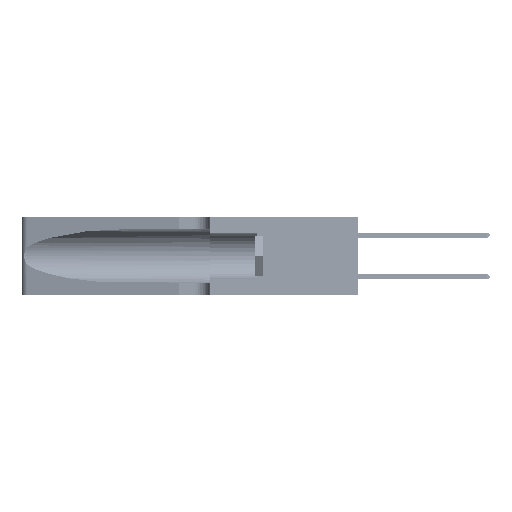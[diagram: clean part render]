
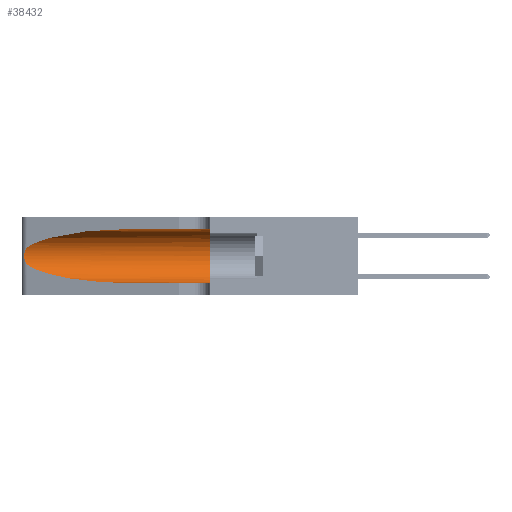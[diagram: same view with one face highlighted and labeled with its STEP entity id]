
A CAD part, left-side view. The second image highlights one B-rep face of the part: STEP entity #38432.
In plain terms, the highlighted cylindrical face has radius 3.308 mm (diameter 6.617 mm), a partial arc.
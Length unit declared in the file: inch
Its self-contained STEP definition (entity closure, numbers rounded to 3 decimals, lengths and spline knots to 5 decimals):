
#1168 = ORIENTED_EDGE ( 'NONE', *, *, #25749, .F. ) ;
#1344 = ORIENTED_EDGE ( 'NONE', *, *, #44045, .T. ) ;
#1497 = CARTESIAN_POINT ( 'NONE',  ( 0.1305, 0.35, 0.185 ) ) ;
#2824 = VERTEX_POINT ( 'NONE', #26665 ) ;
#3456 = CARTESIAN_POINT ( 'NONE',  ( 0.26075, 1.23896, 0.19203 ) ) ;
#3629 = CARTESIAN_POINT ( 'NONE',  ( 0.25487, 1.22718, 0.14631 ) ) ;
#4826 = VERTEX_POINT ( 'NONE', #18742 ) ;
#5212 = CARTESIAN_POINT ( 'NONE',  ( 0.1305, 1.61858, 0.05475 ) ) ;
#5369 = CARTESIAN_POINT ( 'NONE',  ( 0.1305, 0.72297, 0.31525 ) ) ;
#5439 = ORIENTED_EDGE ( 'NONE', *, *, #52243, .T. ) ;
#5553 = CARTESIAN_POINT ( 'NONE',  ( 0.25487, 1.22718, 0.22369 ) ) ;
#5779 = DIRECTION ( 'NONE',  ( 0., 0., 1. ) ) ;
#7472 = VERTEX_POINT ( 'NONE', #21529 ) ;
#7642 = CARTESIAN_POINT ( 'NONE',  ( 0.1305, 0.72297, 0.05475 ) ) ;
#7710 = CARTESIAN_POINT ( 'NONE',  ( 0.26017, 1.23833, 0.17102 ) ) ;
#7958 = DIRECTION ( 'NONE',  ( 0., -1., 0. ) ) ;
#9101 = VERTEX_POINT ( 'NONE', #34016 ) ;
#9995 = DIRECTION ( 'NONE',  ( 0., 0., -1. ) ) ;
#9997 = VECTOR ( 'NONE', #7958, 39.37008 ) ;
#11844 = CARTESIAN_POINT ( 'NONE',  ( 0.25789, 1.23486, 0.15765 ) ) ;
#12841 = VERTEX_POINT ( 'NONE', #13095 ) ;
#13095 = CARTESIAN_POINT ( 'NONE',  ( 0.25487, 1.22718, 0.22369 ) ) ;
#16046 = CARTESIAN_POINT ( 'NONE',  ( 0.25555, 1.22993, 0.14849 ) ) ;
#18019 = CYLINDRICAL_SURFACE ( 'NONE', #38049, 0.13025 ) ;
#18705 = EDGE_CURVE ( 'NONE', #9101, #7472, #33347, .T. ) ;
#18742 = CARTESIAN_POINT ( 'NONE',  ( 0.25487, 1.22718, 0.14631 ) ) ;
#20325 = CARTESIAN_POINT ( 'NONE',  ( 0.18966, 0.96281, 0.05475 ) ) ;
#21442 = EDGE_LOOP ( 'NONE', ( #5439, #1344, #38152, #42464, #42729, #1168 ) ) ;
#21529 = CARTESIAN_POINT ( 'NONE',  ( 0.1305, 0.35, 0.05475 ) ) ;
#21897 = DIRECTION ( 'NONE',  ( 0., -1., 0. ) ) ;
#22286 = CARTESIAN_POINT ( 'NONE',  ( 0.1305, 1.61858, 0.185 ) ) ;
#22339 = VECTOR ( 'NONE', #21897, 39.37008 ) ;
#24150 = CARTESIAN_POINT ( 'NONE',  ( 0.25787, 1.23484, 0.2124 ) ) ;
#25749 = EDGE_CURVE ( 'NONE', #2824, #9101, #52458, .T. ) ;
#26665 = CARTESIAN_POINT ( 'NONE',  ( 0.1305, 0.72297, 0.31525 ) ) ;
#28325 = CARTESIAN_POINT ( 'NONE',  ( 0.26018, 1.23835, 0.19895 ) ) ;
#29240 = AXIS2_PLACEMENT_3D ( 'NONE', #1497, #30591, #5779 ) ;
#30384 = CARTESIAN_POINT ( 'NONE',  ( 0.2373, 1.15595, 0.28018 ) ) ;
#30591 = DIRECTION ( 'NONE',  ( 0., 1., 0. ) ) ;
#32470 = CARTESIAN_POINT ( 'NONE',  ( 0.26075, 1.23896, 0.178 ) ) ;
#33347 = CIRCLE ( 'NONE', #29240, 0.13025 ) ;
#33350 = LINE ( 'NONE', #5212, #22339 ) ;
#34016 = CARTESIAN_POINT ( 'NONE',  ( 0.1305, 0.35, 0.31525 ) ) ;
#34845 = VERTEX_POINT ( 'NONE', #7642 ) ;
#36608 = CARTESIAN_POINT ( 'NONE',  ( 0.2373, 1.15595, 0.08982 ) ) ;
#36633 = CARTESIAN_POINT ( 'NONE',  ( 0.25856, 1.23593, 0.16098 ) ) ;
#36891 = CARTESIAN_POINT ( 'NONE',  ( 0.1305, 1.61858, 0.31525 ) ) ;
#37208 =( BOUNDED_CURVE ( )  B_SPLINE_CURVE ( 3, ( #5369, #42616, #30384, #5553 ),
 .UNSPECIFIED., .F., .F. ) 
 B_SPLINE_CURVE_WITH_KNOTS ( ( 4, 4 ),
 ( 1.5708, 2.84003 ),
 .UNSPECIFIED. ) 
 CURVE ( )  GEOMETRIC_REPRESENTATION_ITEM ( )  RATIONAL_B_SPLINE_CURVE ( ( 1., 0.87, 0.87, 1. ) ) 
 REPRESENTATION_ITEM ( '' )  );
#38049 = AXIS2_PLACEMENT_3D ( 'NONE', #22286, #38924, #9995 ) ;
#38152 = ORIENTED_EDGE ( 'NONE', *, *, #48144, .T. ) ;
#38432 = ADVANCED_FACE ( 'NONE', ( #41263 ), #18019, .F. ) ;
#38924 = DIRECTION ( 'NONE',  ( 0., -1., 0. ) ) ;
#40365 =( BOUNDED_CURVE ( )  B_SPLINE_CURVE ( 3, ( #3629, #36608, #20325, #49110 ),
 .UNSPECIFIED., .F., .F. ) 
 B_SPLINE_CURVE_WITH_KNOTS ( ( 4, 4 ),
 ( 3.44316, 4.71239 ),
 .UNSPECIFIED. ) 
 CURVE ( )  GEOMETRIC_REPRESENTATION_ITEM ( )  RATIONAL_B_SPLINE_CURVE ( ( 1., 0.87, 0.87, 1. ) ) 
 REPRESENTATION_ITEM ( '' )  );
#40417 = CARTESIAN_POINT ( 'NONE',  ( 0.25555, 1.22994, 0.2215 ) ) ;
#40755 = CARTESIAN_POINT ( 'NONE',  ( 0.25639, 1.23186, 0.15144 ) ) ;
#41263 = FACE_OUTER_BOUND ( 'NONE', #21442, .T. ) ;
#42225 = B_SPLINE_CURVE_WITH_KNOTS ( 'NONE', 3,
 ( #44672, #40417, #48772, #24150, #52842, #28325, #3456, #32470, #7710, #36633, #11844, #40755, #16046, #44842 ),
 .UNSPECIFIED., .F., .F.,
 ( 4, 2, 2, 2, 2, 2, 4 ),
 ( 0., 0.00027, 0.00053, 0.00107, 0.0016, 0.00187, 0.00214 ),
 .UNSPECIFIED. ) ;
#42464 = ORIENTED_EDGE ( 'NONE', *, *, #45060, .T. ) ;
#42616 = CARTESIAN_POINT ( 'NONE',  ( 0.18966, 0.96281, 0.31525 ) ) ;
#42729 = ORIENTED_EDGE ( 'NONE', *, *, #18705, .F. ) ;
#44045 = EDGE_CURVE ( 'NONE', #12841, #4826, #42225, .T. ) ;
#44672 = CARTESIAN_POINT ( 'NONE',  ( 0.25487, 1.22718, 0.22369 ) ) ;
#44842 = CARTESIAN_POINT ( 'NONE',  ( 0.25487, 1.22718, 0.14631 ) ) ;
#45060 = EDGE_CURVE ( 'NONE', #34845, #7472, #33350, .T. ) ;
#48144 = EDGE_CURVE ( 'NONE', #4826, #34845, #40365, .T. ) ;
#48772 = CARTESIAN_POINT ( 'NONE',  ( 0.25639, 1.23184, 0.21858 ) ) ;
#49110 = CARTESIAN_POINT ( 'NONE',  ( 0.1305, 0.72297, 0.05475 ) ) ;
#52243 = EDGE_CURVE ( 'NONE', #2824, #12841, #37208, .T. ) ;
#52458 = LINE ( 'NONE', #36891, #9997 ) ;
#52842 = CARTESIAN_POINT ( 'NONE',  ( 0.25854, 1.2359, 0.20912 ) ) ;
